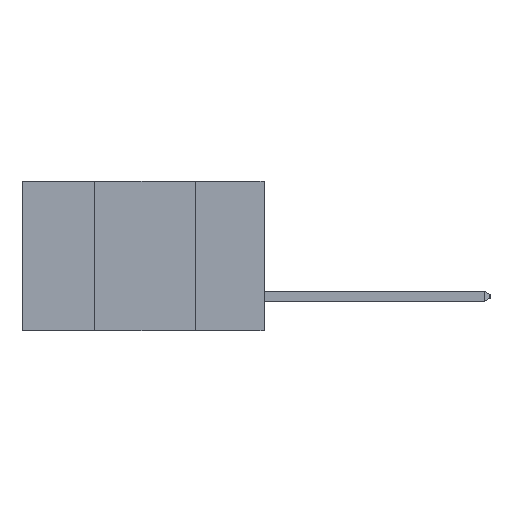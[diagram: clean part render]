
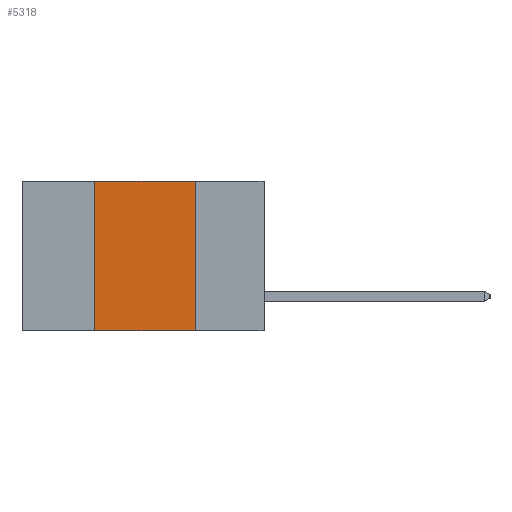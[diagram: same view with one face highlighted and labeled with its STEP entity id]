
A CAD part, left-side view. The second image highlights one B-rep face of the part: STEP entity #5318.
In plain terms, the highlighted planar face has unit normal (-1, 0, 0).
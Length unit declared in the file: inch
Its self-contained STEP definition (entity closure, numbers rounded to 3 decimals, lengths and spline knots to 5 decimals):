
#956 = EDGE_CURVE ( 'NONE', #5855, #8321, #8993, .T. ) ;
#1218 = VECTOR ( 'NONE', #2988, 39.37008 ) ;
#1305 = CARTESIAN_POINT ( 'NONE',  ( 0., 0.17, -0.37 ) ) ;
#1384 = EDGE_LOOP ( 'NONE', ( #5456, #1620, #8514, #5014 ) ) ;
#1428 = DIRECTION ( 'NONE',  ( 0., 0., 1. ) ) ;
#1620 = ORIENTED_EDGE ( 'NONE', *, *, #956, .F. ) ;
#2722 = VECTOR ( 'NONE', #6722, 39.37008 ) ;
#2952 = AXIS2_PLACEMENT_3D ( 'NONE', #11698, #10106, #4789 ) ;
#2988 = DIRECTION ( 'NONE',  ( 0., -1., 0. ) ) ;
#3549 = EDGE_CURVE ( 'NONE', #8321, #4489, #9971, .T. ) ;
#4489 = VERTEX_POINT ( 'NONE', #1305 ) ;
#4789 = DIRECTION ( 'NONE',  ( 0., 0., -1. ) ) ;
#5014 = ORIENTED_EDGE ( 'NONE', *, *, #5823, .T. ) ;
#5318 = ADVANCED_FACE ( 'NONE', ( #8593 ), #5778, .F. ) ;
#5429 = CARTESIAN_POINT ( 'NONE',  ( 0., 0.6, 0. ) ) ;
#5456 = ORIENTED_EDGE ( 'NONE', *, *, #3549, .F. ) ;
#5778 = PLANE ( 'NONE',  #2952 ) ;
#5823 = EDGE_CURVE ( 'NONE', #8915, #4489, #6450, .T. ) ;
#5855 = VERTEX_POINT ( 'NONE', #10354 ) ;
#5915 = CARTESIAN_POINT ( 'NONE',  ( 0., 0.6, -0.37 ) ) ;
#6450 = LINE ( 'NONE', #5915, #1218 ) ;
#6457 = VECTOR ( 'NONE', #9133, 39.37008 ) ;
#6722 = DIRECTION ( 'NONE',  ( 0., 0., -1. ) ) ;
#6765 = LINE ( 'NONE', #8054, #11205 ) ;
#7217 = CARTESIAN_POINT ( 'NONE',  ( 0., 0.17, -0.37 ) ) ;
#7983 = CARTESIAN_POINT ( 'NONE',  ( 0., 0.42, -0.37 ) ) ;
#8054 = CARTESIAN_POINT ( 'NONE',  ( 0., 0.42, -0.37 ) ) ;
#8321 = VERTEX_POINT ( 'NONE', #10013 ) ;
#8514 = ORIENTED_EDGE ( 'NONE', *, *, #11500, .F. ) ;
#8593 = FACE_OUTER_BOUND ( 'NONE', #1384, .T. ) ;
#8915 = VERTEX_POINT ( 'NONE', #7983 ) ;
#8993 = LINE ( 'NONE', #5429, #6457 ) ;
#9133 = DIRECTION ( 'NONE',  ( 0., -1., 0. ) ) ;
#9971 = LINE ( 'NONE', #7217, #2722 ) ;
#10013 = CARTESIAN_POINT ( 'NONE',  ( 0., 0.17, 0. ) ) ;
#10106 = DIRECTION ( 'NONE',  ( 1., 0., 0. ) ) ;
#10354 = CARTESIAN_POINT ( 'NONE',  ( 0., 0.42, 0. ) ) ;
#11205 = VECTOR ( 'NONE', #1428, 39.37008 ) ;
#11500 = EDGE_CURVE ( 'NONE', #8915, #5855, #6765, .T. ) ;
#11698 = CARTESIAN_POINT ( 'NONE',  ( 0., 0.6, 0. ) ) ;
